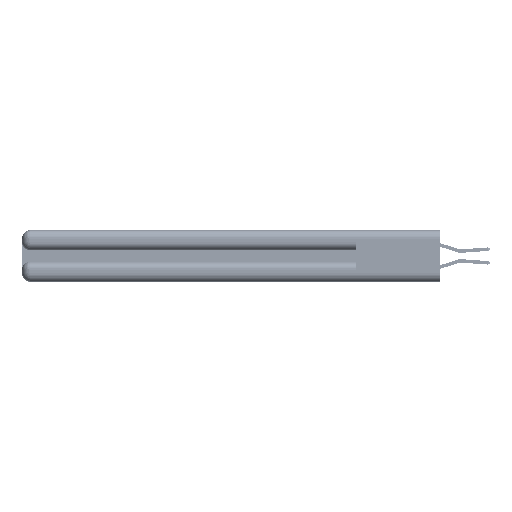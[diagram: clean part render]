
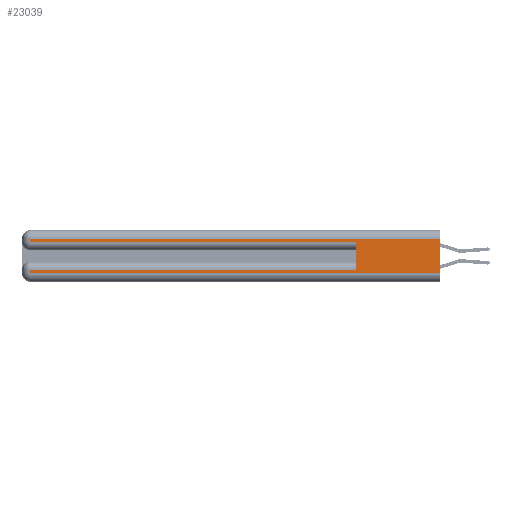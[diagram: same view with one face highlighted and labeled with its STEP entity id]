
A CAD part, left-side view. The second image highlights one B-rep face of the part: STEP entity #23039.
In plain terms, the highlighted planar face has unit normal (-1, 0, 0).
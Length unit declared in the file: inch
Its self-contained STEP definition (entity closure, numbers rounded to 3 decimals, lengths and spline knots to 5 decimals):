
#449 = CARTESIAN_POINT ( 'NONE',  ( 0., 0., 0.31 ) ) ;
#807 = DIRECTION ( 'NONE',  ( 0., 1., 0. ) ) ;
#877 = ORIENTED_EDGE ( 'NONE', *, *, #7654, .T. ) ;
#1720 = EDGE_CURVE ( 'NONE', #25944, #44347, #6122, .T. ) ;
#2904 = VECTOR ( 'NONE', #30561, 39.37008 ) ;
#4016 = LINE ( 'NONE', #34279, #44316 ) ;
#4668 = CARTESIAN_POINT ( 'NONE',  ( 0., 0., 0.06 ) ) ;
#5567 = CARTESIAN_POINT ( 'NONE',  ( 0., 2.94, 0.37 ) ) ;
#6122 = LINE ( 'NONE', #29421, #31764 ) ;
#6145 = VERTEX_POINT ( 'NONE', #4668 ) ;
#6285 = LINE ( 'NONE', #13770, #46577 ) ;
#6994 = ORIENTED_EDGE ( 'NONE', *, *, #44457, .F. ) ;
#7155 = EDGE_CURVE ( 'NONE', #16988, #25944, #9267, .T. ) ;
#7495 = ORIENTED_EDGE ( 'NONE', *, *, #32072, .T. ) ;
#7654 = EDGE_CURVE ( 'NONE', #8901, #11566, #6285, .T. ) ;
#7703 = ORIENTED_EDGE ( 'NONE', *, *, #1720, .T. ) ;
#8122 = DIRECTION ( 'NONE',  ( 0., 0., -1. ) ) ;
#8869 = VECTOR ( 'NONE', #807, 39.37008 ) ;
#8901 = VERTEX_POINT ( 'NONE', #28682 ) ;
#9267 = LINE ( 'NONE', #5567, #17183 ) ;
#10214 = PLANE ( 'NONE',  #12653 ) ;
#11175 = CARTESIAN_POINT ( 'NONE',  ( 0., 2.94, 0.06 ) ) ;
#11566 = VERTEX_POINT ( 'NONE', #46527 ) ;
#12603 = CARTESIAN_POINT ( 'NONE',  ( 0., 2.94, 0.31 ) ) ;
#12653 = AXIS2_PLACEMENT_3D ( 'NONE', #25891, #38177, #22514 ) ;
#13770 = CARTESIAN_POINT ( 'NONE',  ( 0., 0., 0.085 ) ) ;
#16462 = CARTESIAN_POINT ( 'NONE',  ( 0., 0., 0.37 ) ) ;
#16988 = VERTEX_POINT ( 'NONE', #12603 ) ;
#17183 = VECTOR ( 'NONE', #38621, 39.37008 ) ;
#17836 = DIRECTION ( 'NONE',  ( 0., -1., 0. ) ) ;
#18098 = DIRECTION ( 'NONE',  ( 0., 0., -1. ) ) ;
#19104 = ORIENTED_EDGE ( 'NONE', *, *, #19394, .T. ) ;
#19394 = EDGE_CURVE ( 'NONE', #29244, #6145, #23669, .T. ) ;
#22514 = DIRECTION ( 'NONE',  ( 0., 0., -1. ) ) ;
#23039 = ADVANCED_FACE ( 'NONE', ( #36433 ), #10214, .F. ) ;
#23201 = VECTOR ( 'NONE', #8122, 39.37008 ) ;
#23669 = LINE ( 'NONE', #50039, #2904 ) ;
#25879 = DIRECTION ( 'NONE',  ( 0., 1., 0. ) ) ;
#25891 = CARTESIAN_POINT ( 'NONE',  ( 0., 0., 0.37 ) ) ;
#25944 = VERTEX_POINT ( 'NONE', #30349 ) ;
#26849 = CARTESIAN_POINT ( 'NONE',  ( 0., 0.6, 0.285 ) ) ;
#28682 = CARTESIAN_POINT ( 'NONE',  ( 0., 0.6, 0.085 ) ) ;
#28683 = LINE ( 'NONE', #16462, #23201 ) ;
#29244 = VERTEX_POINT ( 'NONE', #11175 ) ;
#29421 = CARTESIAN_POINT ( 'NONE',  ( 0., 0., 0.285 ) ) ;
#30349 = CARTESIAN_POINT ( 'NONE',  ( 0., 2.94, 0.285 ) ) ;
#30547 = ORIENTED_EDGE ( 'NONE', *, *, #31845, .F. ) ;
#30561 = DIRECTION ( 'NONE',  ( 0., -1., 0. ) ) ;
#31706 = VERTEX_POINT ( 'NONE', #48825 ) ;
#31764 = VECTOR ( 'NONE', #17836, 39.37008 ) ;
#31845 = EDGE_CURVE ( 'NONE', #8901, #44347, #38690, .T. ) ;
#32072 = EDGE_CURVE ( 'NONE', #31706, #16988, #45480, .T. ) ;
#33927 = DIRECTION ( 'NONE',  ( 0., 0., 1. ) ) ;
#34095 = CARTESIAN_POINT ( 'NONE',  ( 0., 0.6, 0.145 ) ) ;
#34279 = CARTESIAN_POINT ( 'NONE',  ( 0., 2.94, 0.37 ) ) ;
#36433 = FACE_OUTER_BOUND ( 'NONE', #42508, .T. ) ;
#38177 = DIRECTION ( 'NONE',  ( 1., 0., 0. ) ) ;
#38621 = DIRECTION ( 'NONE',  ( 0., 0., -1. ) ) ;
#38662 = ORIENTED_EDGE ( 'NONE', *, *, #46816, .T. ) ;
#38690 = LINE ( 'NONE', #34095, #47904 ) ;
#41659 = ORIENTED_EDGE ( 'NONE', *, *, #7155, .T. ) ;
#42508 = EDGE_LOOP ( 'NONE', ( #6994, #7495, #41659, #7703, #30547, #877, #38662, #19104 ) ) ;
#44316 = VECTOR ( 'NONE', #18098, 39.37008 ) ;
#44347 = VERTEX_POINT ( 'NONE', #26849 ) ;
#44457 = EDGE_CURVE ( 'NONE', #31706, #6145, #28683, .T. ) ;
#45480 = LINE ( 'NONE', #449, #8869 ) ;
#46527 = CARTESIAN_POINT ( 'NONE',  ( 0., 2.94, 0.085 ) ) ;
#46577 = VECTOR ( 'NONE', #25879, 39.37008 ) ;
#46816 = EDGE_CURVE ( 'NONE', #11566, #29244, #4016, .T. ) ;
#47904 = VECTOR ( 'NONE', #33927, 39.37008 ) ;
#48825 = CARTESIAN_POINT ( 'NONE',  ( 0., 0., 0.31 ) ) ;
#50039 = CARTESIAN_POINT ( 'NONE',  ( 0., 0., 0.06 ) ) ;
